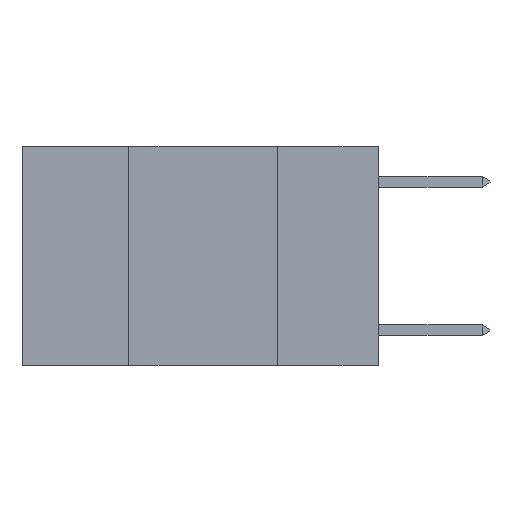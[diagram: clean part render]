
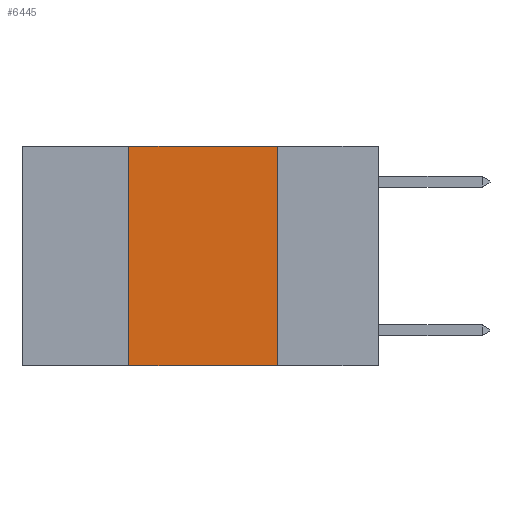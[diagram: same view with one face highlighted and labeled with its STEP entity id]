
A CAD part, left-side view. The second image highlights one B-rep face of the part: STEP entity #6445.
In plain terms, the highlighted planar face has unit normal (-1, 0, 0).
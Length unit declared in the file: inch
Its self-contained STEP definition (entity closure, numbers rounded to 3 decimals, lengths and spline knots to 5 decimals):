
#378 = CARTESIAN_POINT ( 'NONE',  ( 0., 0.6, 0. ) ) ;
#423 = DIRECTION ( 'NONE',  ( 0., 0., -1. ) ) ;
#441 = CARTESIAN_POINT ( 'NONE',  ( 0., 0.42, 0. ) ) ;
#508 = VERTEX_POINT ( 'NONE', #6565 ) ;
#944 = DIRECTION ( 'NONE',  ( 0., 0., 1. ) ) ;
#974 = PLANE ( 'NONE',  #4290 ) ;
#1706 = DIRECTION ( 'NONE',  ( 1., 0., 0. ) ) ;
#1837 = CARTESIAN_POINT ( 'NONE',  ( 0., 0.17, 0. ) ) ;
#2092 = EDGE_CURVE ( 'NONE', #4644, #6209, #6858, .T. ) ;
#2114 = ORIENTED_EDGE ( 'NONE', *, *, #2972, .F. ) ;
#2571 = CARTESIAN_POINT ( 'NONE',  ( 0., 0.42, 0. ) ) ;
#2614 = EDGE_CURVE ( 'NONE', #508, #2783, #5735, .T. ) ;
#2783 = VERTEX_POINT ( 'NONE', #5253 ) ;
#2972 = EDGE_CURVE ( 'NONE', #6209, #508, #2977, .T. ) ;
#2977 = LINE ( 'NONE', #5604, #4813 ) ;
#3505 = DIRECTION ( 'NONE',  ( 0., -1., 0. ) ) ;
#3832 = EDGE_LOOP ( 'NONE', ( #3974, #2114, #7880, #4961 ) ) ;
#3974 = ORIENTED_EDGE ( 'NONE', *, *, #2614, .F. ) ;
#4139 = LINE ( 'NONE', #7241, #8451 ) ;
#4290 = AXIS2_PLACEMENT_3D ( 'NONE', #378, #1706, #423 ) ;
#4366 = CARTESIAN_POINT ( 'NONE',  ( 0., 0.42, -0.37 ) ) ;
#4644 = VERTEX_POINT ( 'NONE', #4366 ) ;
#4813 = VECTOR ( 'NONE', #8298, 39.37008 ) ;
#4961 = ORIENTED_EDGE ( 'NONE', *, *, #6794, .T. ) ;
#5253 = CARTESIAN_POINT ( 'NONE',  ( 0., 0.17, -0.37 ) ) ;
#5604 = CARTESIAN_POINT ( 'NONE',  ( 0., 0.6, 0. ) ) ;
#5735 = LINE ( 'NONE', #1837, #7587 ) ;
#5920 = VECTOR ( 'NONE', #944, 39.37008 ) ;
#6209 = VERTEX_POINT ( 'NONE', #2571 ) ;
#6295 = FACE_OUTER_BOUND ( 'NONE', #3832, .T. ) ;
#6445 = ADVANCED_FACE ( 'NONE', ( #6295 ), #974, .F. ) ;
#6552 = DIRECTION ( 'NONE',  ( 0., 0., -1. ) ) ;
#6565 = CARTESIAN_POINT ( 'NONE',  ( 0., 0.17, 0. ) ) ;
#6794 = EDGE_CURVE ( 'NONE', #4644, #2783, #4139, .T. ) ;
#6858 = LINE ( 'NONE', #441, #5920 ) ;
#7241 = CARTESIAN_POINT ( 'NONE',  ( 0., 0.6, -0.37 ) ) ;
#7587 = VECTOR ( 'NONE', #6552, 39.37008 ) ;
#7880 = ORIENTED_EDGE ( 'NONE', *, *, #2092, .F. ) ;
#8298 = DIRECTION ( 'NONE',  ( 0., -1., 0. ) ) ;
#8451 = VECTOR ( 'NONE', #3505, 39.37008 ) ;
